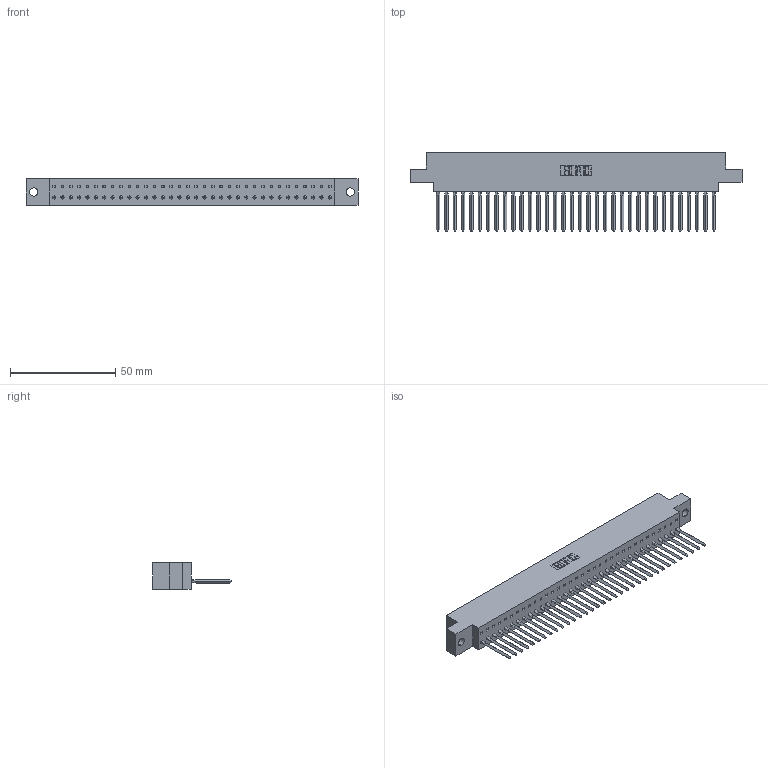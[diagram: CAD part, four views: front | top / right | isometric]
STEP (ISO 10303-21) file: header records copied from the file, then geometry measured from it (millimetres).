
FILE_DESCRIPTION (( 'STEP AP203' ), '1' );
FILE_NAME ('317-034-541-604.STEP', '2020-02-27T21:49:09', ( '' ), ( '' ), 'SwSTEP 2.0', 'SolidWorks 2016', '' );
FILE_SCHEMA (( 'CONFIG_CONTROL_DESIGN' ));
Length unit declared in the file: inch
Products named in the file (3): 317-034-541-604; 317 Part_.156 Dia - TH; 317-290-002_541
Assembly tree (35 placements, depth 2):
  317-034-541-604
    317 Part_.156 Dia - TH
    317-290-002_541  x34
Bounding box: 157.43 x 37.34 x 12.7 mm (x, y, z)
Volume: 25195.9 mm3; surface area: 35154.7 mm2
Topology: 35 solids, 35 shells, 5270 faces, 15031 edges, 9770 vertices
Faces by surface type: plane 4274, cylinder 860, bspline 136
Entity records: 50726 total; most frequent: CARTESIAN_POINT 9655, ORIENTED_EDGE 8942, DIRECTION 7339, EDGE_CURVE 4471, LINE 4107, VECTOR 4107, VERTEX_POINT 2972, AXIS2_PLACEMENT_3D 1616
